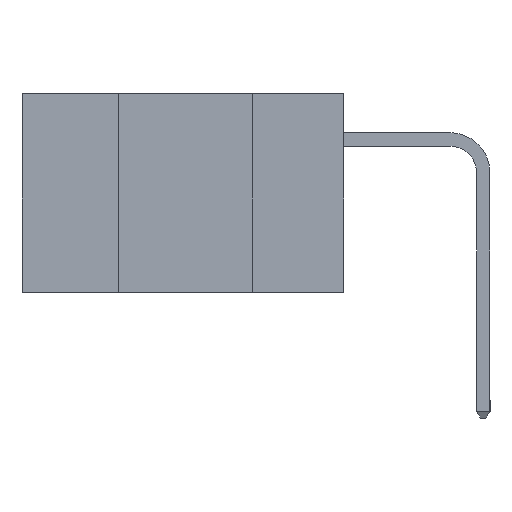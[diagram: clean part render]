
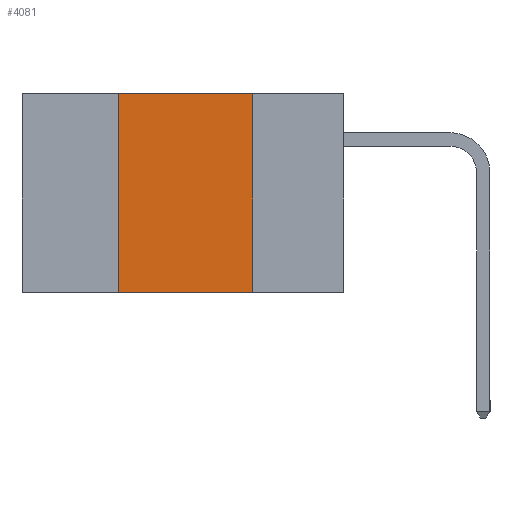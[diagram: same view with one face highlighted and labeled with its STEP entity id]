
A CAD part, left-side view. The second image highlights one B-rep face of the part: STEP entity #4081.
In plain terms, the highlighted planar face has unit normal (-1, 0, 0).
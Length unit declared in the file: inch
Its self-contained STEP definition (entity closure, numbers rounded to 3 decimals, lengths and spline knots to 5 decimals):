
#99 = AXIS2_PLACEMENT_3D ( 'NONE', #10540, #7762, #7213 ) ;
#181 = VECTOR ( 'NONE', #639, 39.37008 ) ;
#320 = VECTOR ( 'NONE', #3666, 39.37008 ) ;
#594 = VECTOR ( 'NONE', #7955, 39.37008 ) ;
#639 = DIRECTION ( 'NONE',  ( 0., -1., 0. ) ) ;
#860 = PLANE ( 'NONE',  #99 ) ;
#1463 = EDGE_CURVE ( 'NONE', #8654, #10191, #7017, .T. ) ;
#1783 = ORIENTED_EDGE ( 'NONE', *, *, #1463, .F. ) ;
#1810 = ORIENTED_EDGE ( 'NONE', *, *, #13654, .T. ) ;
#2490 = CARTESIAN_POINT ( 'NONE',  ( 0., 0.6, -0.37 ) ) ;
#2980 = LINE ( 'NONE', #15023, #594 ) ;
#3250 = CARTESIAN_POINT ( 'NONE',  ( 0., 0.17, -0.37 ) ) ;
#3305 = CARTESIAN_POINT ( 'NONE',  ( 0., 0.17, 0. ) ) ;
#3666 = DIRECTION ( 'NONE',  ( 0., -1., 0. ) ) ;
#3681 = LINE ( 'NONE', #8957, #181 ) ;
#3849 = VECTOR ( 'NONE', #5782, 39.37008 ) ;
#4081 = ADVANCED_FACE ( 'NONE', ( #9387 ), #860, .F. ) ;
#4356 = CARTESIAN_POINT ( 'NONE',  ( 0., 0.42, -0.37 ) ) ;
#5782 = DIRECTION ( 'NONE',  ( 0., 0., 1. ) ) ;
#7017 = LINE ( 'NONE', #8916, #3849 ) ;
#7139 = CARTESIAN_POINT ( 'NONE',  ( 0., 0.42, 0. ) ) ;
#7213 = DIRECTION ( 'NONE',  ( 0., 0., -1. ) ) ;
#7320 = EDGE_CURVE ( 'NONE', #10191, #11055, #3681, .T. ) ;
#7762 = DIRECTION ( 'NONE',  ( 1., 0., 0. ) ) ;
#7955 = DIRECTION ( 'NONE',  ( 0., 0., -1. ) ) ;
#8111 = EDGE_CURVE ( 'NONE', #11055, #12979, #2980, .T. ) ;
#8403 = EDGE_LOOP ( 'NONE', ( #8918, #13650, #1783, #1810 ) ) ;
#8654 = VERTEX_POINT ( 'NONE', #4356 ) ;
#8916 = CARTESIAN_POINT ( 'NONE',  ( 0., 0.42, -0.37 ) ) ;
#8918 = ORIENTED_EDGE ( 'NONE', *, *, #8111, .F. ) ;
#8957 = CARTESIAN_POINT ( 'NONE',  ( 0., 0.6, 0. ) ) ;
#9387 = FACE_OUTER_BOUND ( 'NONE', #8403, .T. ) ;
#9456 = LINE ( 'NONE', #2490, #320 ) ;
#10191 = VERTEX_POINT ( 'NONE', #7139 ) ;
#10540 = CARTESIAN_POINT ( 'NONE',  ( 0., 0.6, 0. ) ) ;
#11055 = VERTEX_POINT ( 'NONE', #3305 ) ;
#12979 = VERTEX_POINT ( 'NONE', #3250 ) ;
#13650 = ORIENTED_EDGE ( 'NONE', *, *, #7320, .F. ) ;
#13654 = EDGE_CURVE ( 'NONE', #8654, #12979, #9456, .T. ) ;
#15023 = CARTESIAN_POINT ( 'NONE',  ( 0., 0.17, -0.37 ) ) ;
